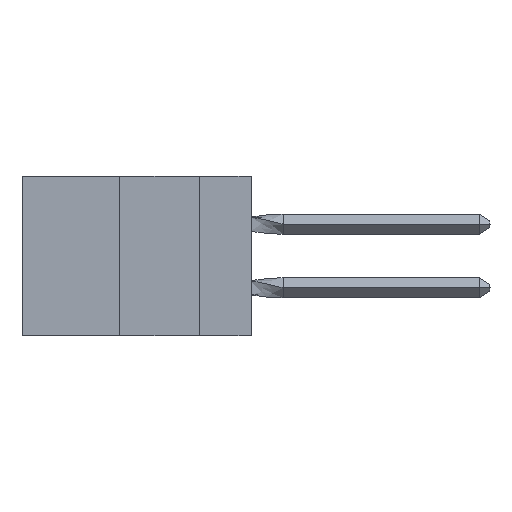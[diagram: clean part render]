
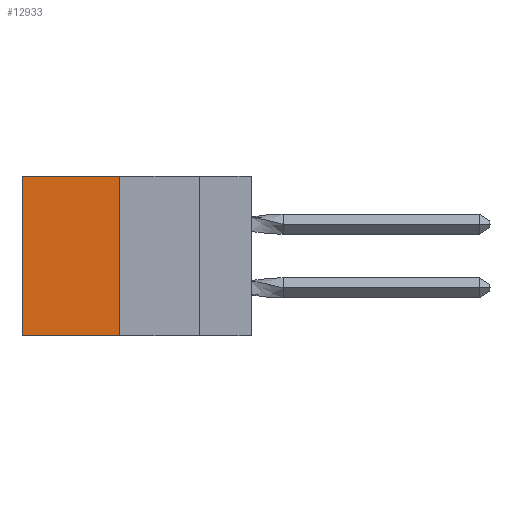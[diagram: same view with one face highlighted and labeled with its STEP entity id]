
A CAD part, left-side view. The second image highlights one B-rep face of the part: STEP entity #12933.
In plain terms, the highlighted planar face has unit normal (-1, 0, 0).
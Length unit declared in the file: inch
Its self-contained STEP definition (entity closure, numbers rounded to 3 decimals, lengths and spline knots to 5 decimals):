
#366 = CARTESIAN_POINT ( 'NONE',  ( 0.305, 0.72, -0.5 ) ) ;
#1903 = CARTESIAN_POINT ( 'NONE',  ( 0.305, 0.413, 0. ) ) ;
#2029 = CARTESIAN_POINT ( 'NONE',  ( 0.305, 0.413, -0.5 ) ) ;
#3038 = LINE ( 'NONE', #27957, #22048 ) ;
#3236 = VERTEX_POINT ( 'NONE', #24214 ) ;
#6312 = ORIENTED_EDGE ( 'NONE', *, *, #19828, .F. ) ;
#9341 = VECTOR ( 'NONE', #33404, 39.37008 ) ;
#9502 = EDGE_LOOP ( 'NONE', ( #27630, #16604, #6312, #37542 ) ) ;
#11686 = LINE ( 'NONE', #11766, #14415 ) ;
#11766 = CARTESIAN_POINT ( 'NONE',  ( 0.305, 0.413, -0.5 ) ) ;
#12933 = ADVANCED_FACE ( 'NONE', ( #26815 ), #29346, .F. ) ;
#13966 = VECTOR ( 'NONE', #25184, 39.37008 ) ;
#14415 = VECTOR ( 'NONE', #26096, 39.37008 ) ;
#14794 = CARTESIAN_POINT ( 'NONE',  ( 0.305, 0.413, -0.5 ) ) ;
#14921 = CARTESIAN_POINT ( 'NONE',  ( 0.305, 0.413, 0. ) ) ;
#15055 = DIRECTION ( 'NONE',  ( 1., 0., 0. ) ) ;
#16604 = ORIENTED_EDGE ( 'NONE', *, *, #30973, .F. ) ;
#18397 = EDGE_CURVE ( 'NONE', #26816, #18695, #29383, .T. ) ;
#18695 = VERTEX_POINT ( 'NONE', #34696 ) ;
#19828 = EDGE_CURVE ( 'NONE', #26816, #3236, #22456, .T. ) ;
#20190 = AXIS2_PLACEMENT_3D ( 'NONE', #14794, #15055, #26726 ) ;
#22048 = VECTOR ( 'NONE', #36103, 39.37008 ) ;
#22456 = LINE ( 'NONE', #2029, #9341 ) ;
#24214 = CARTESIAN_POINT ( 'NONE',  ( 0.305, 0.413, -0.5 ) ) ;
#25184 = DIRECTION ( 'NONE',  ( 0., 1., 0. ) ) ;
#26096 = DIRECTION ( 'NONE',  ( 0., 1., 0. ) ) ;
#26726 = DIRECTION ( 'NONE',  ( 0., 0., -1. ) ) ;
#26815 = FACE_OUTER_BOUND ( 'NONE', #9502, .T. ) ;
#26816 = VERTEX_POINT ( 'NONE', #14921 ) ;
#27630 = ORIENTED_EDGE ( 'NONE', *, *, #31917, .T. ) ;
#27957 = CARTESIAN_POINT ( 'NONE',  ( 0.305, 0.72, -0.5 ) ) ;
#29346 = PLANE ( 'NONE',  #20190 ) ;
#29383 = LINE ( 'NONE', #1903, #13966 ) ;
#30973 = EDGE_CURVE ( 'NONE', #3236, #34933, #11686, .T. ) ;
#31917 = EDGE_CURVE ( 'NONE', #18695, #34933, #3038, .T. ) ;
#33404 = DIRECTION ( 'NONE',  ( 0., 0., -1. ) ) ;
#34696 = CARTESIAN_POINT ( 'NONE',  ( 0.305, 0.72, 0. ) ) ;
#34933 = VERTEX_POINT ( 'NONE', #366 ) ;
#36103 = DIRECTION ( 'NONE',  ( 0., 0., -1. ) ) ;
#37542 = ORIENTED_EDGE ( 'NONE', *, *, #18397, .T. ) ;
